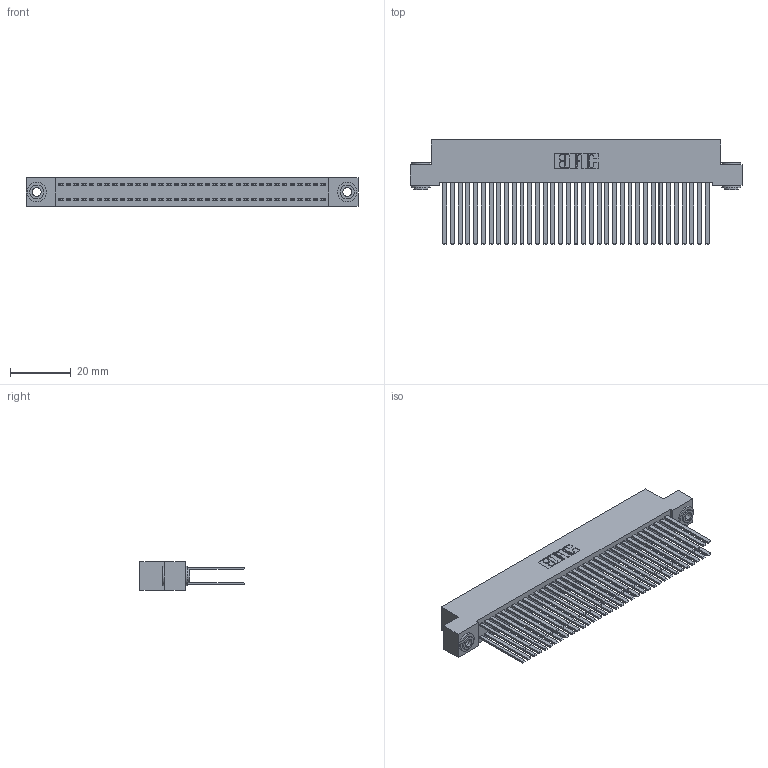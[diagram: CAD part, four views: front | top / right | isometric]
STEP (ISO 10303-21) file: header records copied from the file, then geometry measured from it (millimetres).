
FILE_DESCRIPTION (( 'STEP AP203' ), '1' );
FILE_NAME ('392-070-544-203.STEP', '2018-08-17T23:34:11', ( '' ), ( '' ), 'SwSTEP 2.0', 'SolidWorks 2016', '' );
FILE_SCHEMA (( 'CONFIG_CONTROL_DESIGN' ));
Length unit declared in the file: inch
Products named in the file (4): 342 Part_.156 TH; 345-292-001_345-293-144; 342-250-002_345-250-002-102; 392-070-544-203
Assembly tree (73 placements, depth 2):
  392-070-544-203
    342 Part_.156 TH
    345-292-001_345-293-144  x70
    342-250-002_345-250-002-102  x2
Bounding box: 109.22 x 34.3 x 9.4 mm (x, y, z)
Volume: 10784.4 mm3; surface area: 20313.3 mm2
Topology: 73 solids, 73 shells, 3368 faces, 9965 edges, 6546 vertices
Faces by surface type: plane 2316, cylinder 1044, cone 8
Entity records: 23756 total; most frequent: CARTESIAN_POINT 3917, ORIENTED_EDGE 3846, DIRECTION 3389, EDGE_CURVE 1923, LINE 1775, VECTOR 1775, VERTEX_POINT 1278, AXIS2_PLACEMENT_3D 807
